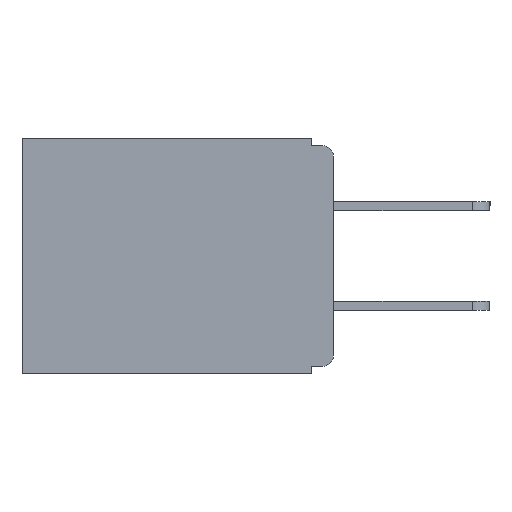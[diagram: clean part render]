
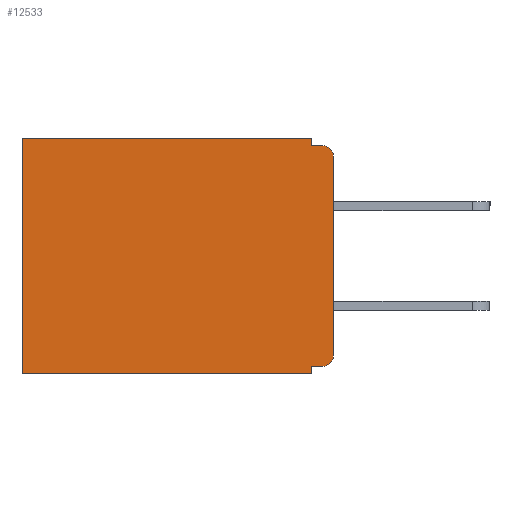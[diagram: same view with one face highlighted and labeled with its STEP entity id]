
A CAD part, left-side view. The second image highlights one B-rep face of the part: STEP entity #12533.
In plain terms, the highlighted planar face has unit normal (-1, 0, 0).
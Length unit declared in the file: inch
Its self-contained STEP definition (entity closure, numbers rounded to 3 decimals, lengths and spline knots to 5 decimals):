
#558 = DIRECTION ( 'NONE',  ( -1., 0., 0. ) ) ;
#815 = CARTESIAN_POINT ( 'NONE',  ( 0.3, 0.015, -0.32 ) ) ;
#1211 = VERTEX_POINT ( 'NONE', #11749 ) ;
#1323 = CARTESIAN_POINT ( 'NONE',  ( 0.3, 0., -0.305 ) ) ;
#1974 = ORIENTED_EDGE ( 'NONE', *, *, #8723, .T. ) ;
#1998 = CARTESIAN_POINT ( 'NONE',  ( 0.3, 0.437, -0.33 ) ) ;
#2620 = VERTEX_POINT ( 'NONE', #1323 ) ;
#2772 = EDGE_CURVE ( 'NONE', #24915, #1211, #26453, .T. ) ;
#2794 = VERTEX_POINT ( 'NONE', #23877 ) ;
#3504 = DIRECTION ( 'NONE',  ( 0., 1., 0. ) ) ;
#4025 = CARTESIAN_POINT ( 'NONE',  ( 0.3, 0., -0.33 ) ) ;
#5808 = VECTOR ( 'NONE', #3504, 39.37008 ) ;
#6371 = CARTESIAN_POINT ( 'NONE',  ( 0.3, 0.015, -0.305 ) ) ;
#6539 = PLANE ( 'NONE',  #20695 ) ;
#7611 = CARTESIAN_POINT ( 'NONE',  ( 0.3, 0.031, 0. ) ) ;
#8723 = EDGE_CURVE ( 'NONE', #30270, #18163, #19028, .T. ) ;
#8975 = ORIENTED_EDGE ( 'NONE', *, *, #22224, .T. ) ;
#8990 = DIRECTION ( 'NONE',  ( 0., 0., -1. ) ) ;
#9057 = EDGE_CURVE ( 'NONE', #18163, #1211, #21702, .T. ) ;
#9375 = EDGE_CURVE ( 'NONE', #2794, #13190, #10282, .T. ) ;
#9539 = CARTESIAN_POINT ( 'NONE',  ( 0.3, 0., -0.32 ) ) ;
#10282 = LINE ( 'NONE', #11758, #29833 ) ;
#10293 = DIRECTION ( 'NONE',  ( 0., 0., -1. ) ) ;
#10390 = VECTOR ( 'NONE', #21600, 39.37008 ) ;
#10486 = VECTOR ( 'NONE', #10293, 39.37008 ) ;
#10608 = LINE ( 'NONE', #9539, #17620 ) ;
#10636 = ORIENTED_EDGE ( 'NONE', *, *, #9375, .F. ) ;
#11749 = CARTESIAN_POINT ( 'NONE',  ( 0.3, 0.437, -0.33 ) ) ;
#11758 = CARTESIAN_POINT ( 'NONE',  ( 0.3, 0., -0.01 ) ) ;
#11806 = DIRECTION ( 'NONE',  ( 1., 0., 0. ) ) ;
#11841 = ORIENTED_EDGE ( 'NONE', *, *, #13940, .F. ) ;
#12533 = ADVANCED_FACE ( 'NONE', ( #24604 ), #6539, .F. ) ;
#12566 = DIRECTION ( 'NONE',  ( 0., 0., -1. ) ) ;
#12645 = CARTESIAN_POINT ( 'NONE',  ( 0.3, 0.031, -0.33 ) ) ;
#12663 = ORIENTED_EDGE ( 'NONE', *, *, #9057, .T. ) ;
#13190 = VERTEX_POINT ( 'NONE', #30054 ) ;
#13838 = CARTESIAN_POINT ( 'NONE',  ( 0.3, 0., 0. ) ) ;
#13940 = EDGE_CURVE ( 'NONE', #29124, #24915, #28773, .T. ) ;
#14885 = AXIS2_PLACEMENT_3D ( 'NONE', #6371, #24520, #8990 ) ;
#16261 = CIRCLE ( 'NONE', #14885, 0.015 ) ;
#16297 = CARTESIAN_POINT ( 'NONE',  ( 0.3, 0.015, -0.025 ) ) ;
#17163 = VERTEX_POINT ( 'NONE', #32135 ) ;
#17477 = CARTESIAN_POINT ( 'NONE',  ( 0.3, 0.031, 0. ) ) ;
#17620 = VECTOR ( 'NONE', #27479, 39.37008 ) ;
#17955 = DIRECTION ( 'NONE',  ( 0., 0., -1. ) ) ;
#17973 = DIRECTION ( 'NONE',  ( 0., 0., -1. ) ) ;
#18163 = VERTEX_POINT ( 'NONE', #28849 ) ;
#18855 = VECTOR ( 'NONE', #17955, 39.37008 ) ;
#18973 = DIRECTION ( 'NONE',  ( 0., 0., -1. ) ) ;
#19028 = LINE ( 'NONE', #13838, #10390 ) ;
#19891 = VERTEX_POINT ( 'NONE', #815 ) ;
#20695 = AXIS2_PLACEMENT_3D ( 'NONE', #29559, #11806, #29663 ) ;
#21600 = DIRECTION ( 'NONE',  ( 0., 1., 0. ) ) ;
#21631 = ORIENTED_EDGE ( 'NONE', *, *, #29540, .T. ) ;
#21702 = LINE ( 'NONE', #1998, #26774 ) ;
#21999 = EDGE_CURVE ( 'NONE', #17163, #2620, #25547, .T. ) ;
#22164 = VECTOR ( 'NONE', #17973, 39.37008 ) ;
#22224 = EDGE_CURVE ( 'NONE', #17163, #13190, #32490, .T. ) ;
#23877 = CARTESIAN_POINT ( 'NONE',  ( 0.3, 0.031, -0.01 ) ) ;
#23978 = EDGE_CURVE ( 'NONE', #30270, #2794, #24238, .T. ) ;
#24238 = LINE ( 'NONE', #7611, #10486 ) ;
#24520 = DIRECTION ( 'NONE',  ( -1., 0., 0. ) ) ;
#24604 = FACE_OUTER_BOUND ( 'NONE', #31530, .T. ) ;
#24915 = VERTEX_POINT ( 'NONE', #32012 ) ;
#25191 = ORIENTED_EDGE ( 'NONE', *, *, #21999, .F. ) ;
#25547 = LINE ( 'NONE', #30539, #18855 ) ;
#26453 = LINE ( 'NONE', #4025, #5808 ) ;
#26774 = VECTOR ( 'NONE', #12566, 39.37008 ) ;
#27093 = ORIENTED_EDGE ( 'NONE', *, *, #2772, .F. ) ;
#27118 = DIRECTION ( 'NONE',  ( 0., -1., 0. ) ) ;
#27479 = DIRECTION ( 'NONE',  ( 0., 1., 0. ) ) ;
#27867 = ORIENTED_EDGE ( 'NONE', *, *, #23978, .F. ) ;
#28490 = EDGE_CURVE ( 'NONE', #19891, #29124, #10608, .T. ) ;
#28773 = LINE ( 'NONE', #12645, #22164 ) ;
#28849 = CARTESIAN_POINT ( 'NONE',  ( 0.3, 0.437, 0. ) ) ;
#29039 = AXIS2_PLACEMENT_3D ( 'NONE', #16297, #558, #18973 ) ;
#29124 = VERTEX_POINT ( 'NONE', #29829 ) ;
#29540 = EDGE_CURVE ( 'NONE', #19891, #2620, #16261, .T. ) ;
#29559 = CARTESIAN_POINT ( 'NONE',  ( 0.3, 0., -0.33 ) ) ;
#29663 = DIRECTION ( 'NONE',  ( 0., 0., -1. ) ) ;
#29829 = CARTESIAN_POINT ( 'NONE',  ( 0.3, 0.031, -0.32 ) ) ;
#29833 = VECTOR ( 'NONE', #27118, 39.37008 ) ;
#30054 = CARTESIAN_POINT ( 'NONE',  ( 0.3, 0.015, -0.01 ) ) ;
#30270 = VERTEX_POINT ( 'NONE', #17477 ) ;
#30539 = CARTESIAN_POINT ( 'NONE',  ( 0.3, 0., -0.33 ) ) ;
#31530 = EDGE_LOOP ( 'NONE', ( #25191, #8975, #10636, #27867, #1974, #12663, #27093, #11841, #32115, #21631 ) ) ;
#32012 = CARTESIAN_POINT ( 'NONE',  ( 0.3, 0.031, -0.33 ) ) ;
#32115 = ORIENTED_EDGE ( 'NONE', *, *, #28490, .F. ) ;
#32135 = CARTESIAN_POINT ( 'NONE',  ( 0.3, 0., -0.025 ) ) ;
#32490 = CIRCLE ( 'NONE', #29039, 0.015 ) ;
